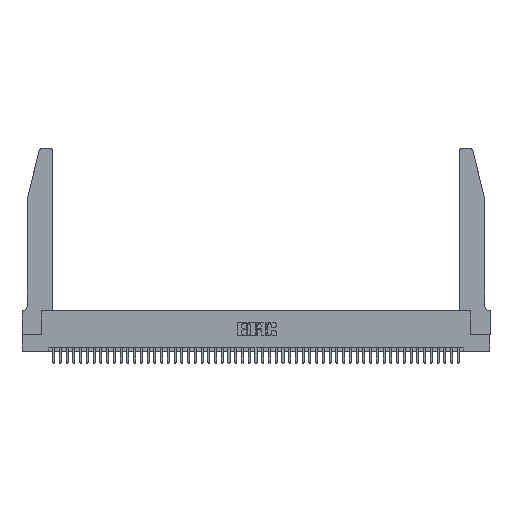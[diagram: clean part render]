
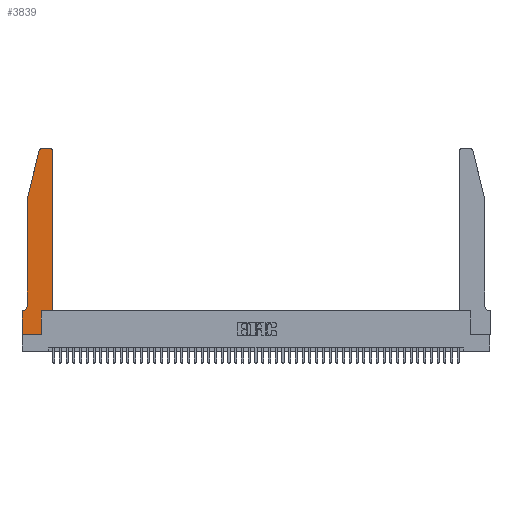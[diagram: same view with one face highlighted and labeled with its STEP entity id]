
A CAD part, top view. The second image highlights one B-rep face of the part: STEP entity #3839.
In plain terms, the highlighted planar face has unit normal (0, 0, 1).
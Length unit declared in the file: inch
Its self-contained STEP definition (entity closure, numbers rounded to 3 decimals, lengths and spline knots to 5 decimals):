
#767 = CARTESIAN_POINT ( 'NONE',  ( 0., 0.35, 0.37 ) ) ;
#1624 = CARTESIAN_POINT ( 'NONE',  ( 0.2865, 0.35, 0.37 ) ) ;
#2075 = DIRECTION ( 'NONE',  ( -1., 0., 0. ) ) ;
#2100 = ORIENTED_EDGE ( 'NONE', *, *, #26147, .T. ) ;
#2151 = VERTEX_POINT ( 'NONE', #36785 ) ;
#2985 = DIRECTION ( 'NONE',  ( 0., 0., 1. ) ) ;
#3839 = ADVANCED_FACE ( 'NONE', ( #9772 ), #24079, .T. ) ;
#4021 = VERTEX_POINT ( 'NONE', #13491 ) ;
#4667 = DIRECTION ( 'NONE',  ( 1., 0., 0. ) ) ;
#4957 = VECTOR ( 'NONE', #39663, 39.37008 ) ;
#6429 = ORIENTED_EDGE ( 'NONE', *, *, #19110, .T. ) ;
#6983 = DIRECTION ( 'NONE',  ( -0.239, -0.971, 0. ) ) ;
#7188 = DIRECTION ( 'NONE',  ( 1., 0., 0. ) ) ;
#8839 = CARTESIAN_POINT ( 'NONE',  ( 0., 0., 0.37 ) ) ;
#9772 = FACE_OUTER_BOUND ( 'NONE', #23497, .T. ) ;
#9953 = CARTESIAN_POINT ( 'NONE',  ( 0.2605, 2.75, 0.37 ) ) ;
#10095 = EDGE_CURVE ( 'NONE', #38060, #24136, #44671, .T. ) ;
#11133 = EDGE_CURVE ( 'NONE', #14017, #25154, #22519, .T. ) ;
#11718 = CARTESIAN_POINT ( 'NONE',  ( 0.0755, 2., 0.37 ) ) ;
#12114 = EDGE_CURVE ( 'NONE', #2151, #45434, #40613, .T. ) ;
#12165 = VECTOR ( 'NONE', #13842, 39.37008 ) ;
#12974 = ORIENTED_EDGE ( 'NONE', *, *, #10095, .T. ) ;
#13117 = CARTESIAN_POINT ( 'NONE',  ( 0.4505, 0.35, 0.37 ) ) ;
#13212 = EDGE_CURVE ( 'NONE', #24136, #14017, #43004, .T. ) ;
#13491 = CARTESIAN_POINT ( 'NONE',  ( 0.25487, 2.72718, 0.37 ) ) ;
#13842 = DIRECTION ( 'NONE',  ( 0., 1., 0. ) ) ;
#13860 = DIRECTION ( 'NONE',  ( -1., 0., 0. ) ) ;
#14017 = VERTEX_POINT ( 'NONE', #13117 ) ;
#14306 = CARTESIAN_POINT ( 'NONE',  ( 0., 0.35, 0.37 ) ) ;
#14472 = CIRCLE ( 'NONE', #18841, 0.03 ) ;
#14804 = CARTESIAN_POINT ( 'NONE',  ( 0., 0., 0.37 ) ) ;
#14909 = VECTOR ( 'NONE', #18362, 39.37008 ) ;
#15136 = CARTESIAN_POINT ( 'NONE',  ( 0.0055, 0.35, 0.37 ) ) ;
#16982 = AXIS2_PLACEMENT_3D ( 'NONE', #41564, #18282, #45454 ) ;
#18093 = ORIENTED_EDGE ( 'NONE', *, *, #18486, .T. ) ;
#18282 = DIRECTION ( 'NONE',  ( 0., 0., 1. ) ) ;
#18362 = DIRECTION ( 'NONE',  ( 0., 1., 0. ) ) ;
#18365 = CARTESIAN_POINT ( 'NONE',  ( 0.0755, 0.35, 0.37 ) ) ;
#18486 = EDGE_CURVE ( 'NONE', #25154, #30610, #14472, .T. ) ;
#18671 = DIRECTION ( 'NONE',  ( 0., -1., 0. ) ) ;
#18841 = AXIS2_PLACEMENT_3D ( 'NONE', #26318, #2985, #30214 ) ;
#18948 = CIRCLE ( 'NONE', #16982, 0.03 ) ;
#19110 = EDGE_CURVE ( 'NONE', #4021, #2151, #48325, .T. ) ;
#19944 = VECTOR ( 'NONE', #38913, 39.37008 ) ;
#20472 = VECTOR ( 'NONE', #13860, 39.37008 ) ;
#20779 = VECTOR ( 'NONE', #18671, 39.37008 ) ;
#22105 = EDGE_CURVE ( 'NONE', #28108, #4021, #18948, .T. ) ;
#22145 = DIRECTION ( 'NONE',  ( -1., 0., 0. ) ) ;
#22519 = LINE ( 'NONE', #41003, #12165 ) ;
#23497 = EDGE_LOOP ( 'NONE', ( #48942, #38131, #6429, #42252, #27689, #2100, #48790, #36115, #12974, #41213, #30946, #18093 ) ) ;
#24079 = PLANE ( 'NONE',  #27550 ) ;
#24136 = VERTEX_POINT ( 'NONE', #1624 ) ;
#25154 = VERTEX_POINT ( 'NONE', #31329 ) ;
#25386 = DIRECTION ( 'NONE',  ( 0., 0., -1. ) ) ;
#26082 = VERTEX_POINT ( 'NONE', #14306 ) ;
#26147 = EDGE_CURVE ( 'NONE', #46450, #26082, #39230, .T. ) ;
#26318 = CARTESIAN_POINT ( 'NONE',  ( 0.4205, 2.72, 0.37 ) ) ;
#26634 = VECTOR ( 'NONE', #6983, 39.37008 ) ;
#27550 = AXIS2_PLACEMENT_3D ( 'NONE', #767, #28002, #4667 ) ;
#27689 = ORIENTED_EDGE ( 'NONE', *, *, #34206, .T. ) ;
#27762 = CIRCLE ( 'NONE', #36510, 0.07 ) ;
#28002 = DIRECTION ( 'NONE',  ( 0., 0., 1. ) ) ;
#28108 = VERTEX_POINT ( 'NONE', #42323 ) ;
#30214 = DIRECTION ( 'NONE',  ( 1., 0., 0. ) ) ;
#30610 = VERTEX_POINT ( 'NONE', #41833 ) ;
#30874 = CARTESIAN_POINT ( 'NONE',  ( 0.0755, 0.42, 0.37 ) ) ;
#30946 = ORIENTED_EDGE ( 'NONE', *, *, #11133, .T. ) ;
#30968 = VERTEX_POINT ( 'NONE', #8839 ) ;
#31329 = CARTESIAN_POINT ( 'NONE',  ( 0.4505, 2.72, 0.37 ) ) ;
#31900 = CARTESIAN_POINT ( 'NONE',  ( 0., 0., 0.37 ) ) ;
#32132 = CARTESIAN_POINT ( 'NONE',  ( 0.2865, 0., 0.37 ) ) ;
#32746 = VECTOR ( 'NONE', #7188, 39.37008 ) ;
#33557 = EDGE_CURVE ( 'NONE', #30610, #28108, #39949, .T. ) ;
#34206 = EDGE_CURVE ( 'NONE', #45434, #46450, #27762, .T. ) ;
#34263 = CARTESIAN_POINT ( 'NONE',  ( 0.0755, 2., 0.37 ) ) ;
#36115 = ORIENTED_EDGE ( 'NONE', *, *, #38233, .T. ) ;
#36510 = AXIS2_PLACEMENT_3D ( 'NONE', #48518, #25386, #2075 ) ;
#36785 = CARTESIAN_POINT ( 'NONE',  ( 0.0755, 2., 0.37 ) ) ;
#37775 = CARTESIAN_POINT ( 'NONE',  ( 0.2865, 0.35, 0.37 ) ) ;
#38060 = VERTEX_POINT ( 'NONE', #32132 ) ;
#38131 = ORIENTED_EDGE ( 'NONE', *, *, #22105, .T. ) ;
#38233 = EDGE_CURVE ( 'NONE', #30968, #38060, #46278, .T. ) ;
#38311 = CARTESIAN_POINT ( 'NONE',  ( 0.4505, 0.35, 0.37 ) ) ;
#38913 = DIRECTION ( 'NONE',  ( 0., -1., 0. ) ) ;
#39230 = LINE ( 'NONE', #18365, #44669 ) ;
#39663 = DIRECTION ( 'NONE',  ( 1., 0., 0. ) ) ;
#39949 = LINE ( 'NONE', #9953, #20472 ) ;
#40613 = LINE ( 'NONE', #11718, #19944 ) ;
#41003 = CARTESIAN_POINT ( 'NONE',  ( 0.4505, 0.35, 0.37 ) ) ;
#41213 = ORIENTED_EDGE ( 'NONE', *, *, #13212, .T. ) ;
#41460 = LINE ( 'NONE', #14804, #20779 ) ;
#41564 = CARTESIAN_POINT ( 'NONE',  ( 0.284, 2.72, 0.37 ) ) ;
#41833 = CARTESIAN_POINT ( 'NONE',  ( 0.4205, 2.75, 0.37 ) ) ;
#42252 = ORIENTED_EDGE ( 'NONE', *, *, #12114, .T. ) ;
#42323 = CARTESIAN_POINT ( 'NONE',  ( 0.284, 2.75, 0.37 ) ) ;
#43004 = LINE ( 'NONE', #38311, #32746 ) ;
#44669 = VECTOR ( 'NONE', #22145, 39.37008 ) ;
#44671 = LINE ( 'NONE', #37775, #14909 ) ;
#45434 = VERTEX_POINT ( 'NONE', #30874 ) ;
#45454 = DIRECTION ( 'NONE',  ( 1., 0., 0. ) ) ;
#45941 = EDGE_CURVE ( 'NONE', #26082, #30968, #41460, .T. ) ;
#46278 = LINE ( 'NONE', #31900, #4957 ) ;
#46450 = VERTEX_POINT ( 'NONE', #15136 ) ;
#48325 = LINE ( 'NONE', #34263, #26634 ) ;
#48518 = CARTESIAN_POINT ( 'NONE',  ( 0.0055, 0.42, 0.37 ) ) ;
#48790 = ORIENTED_EDGE ( 'NONE', *, *, #45941, .T. ) ;
#48942 = ORIENTED_EDGE ( 'NONE', *, *, #33557, .T. ) ;
